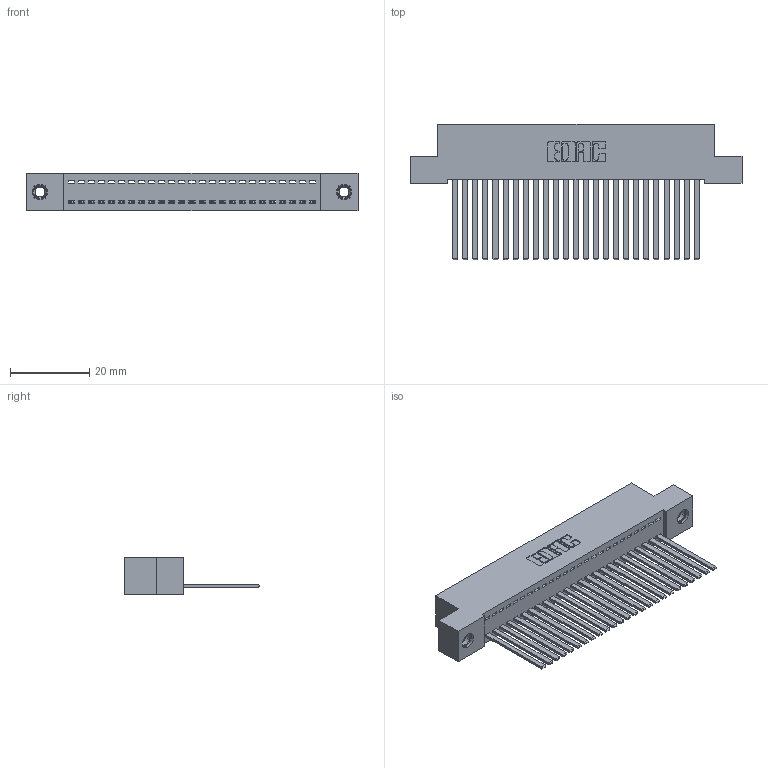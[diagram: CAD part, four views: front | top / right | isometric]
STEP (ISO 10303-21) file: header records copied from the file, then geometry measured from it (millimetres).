
FILE_DESCRIPTION (( 'STEP AP203' ), '1' );
FILE_NAME ('392-025-544-107.STEP', '2019-10-07T10:59:57', ( '' ), ( '' ), 'SwSTEP 2.0', 'SolidWorks 2016', '' );
FILE_SCHEMA (( 'CONFIG_CONTROL_DESIGN' ));
Length unit declared in the file: inch
Products named in the file (4): 342 Part_TI; 345-292-001_345-293-144; 345-250-001_345-250-005-103; 392-025-544-107
Assembly tree (28 placements, depth 2):
  392-025-544-107
    342 Part_TI
    345-292-001_345-293-144  x25
    345-250-001_345-250-005-103  x2
Bounding box: 83.82 x 34.3 x 9.4 mm (x, y, z)
Volume: 7563.6 mm3; surface area: 11645.6 mm2
Topology: 28 solids, 28 shells, 1470 faces, 4385 edges, 2882 vertices
Faces by surface type: plane 1048, cylinder 406, cone 12, torus 4
Entity records: 18352 total; most frequent: CARTESIAN_POINT 3148, ORIENTED_EDGE 3102, DIRECTION 2719, EDGE_CURVE 1551, LINE 1407, VECTOR 1407, VERTEX_POINT 1028, AXIS2_PLACEMENT_3D 656
